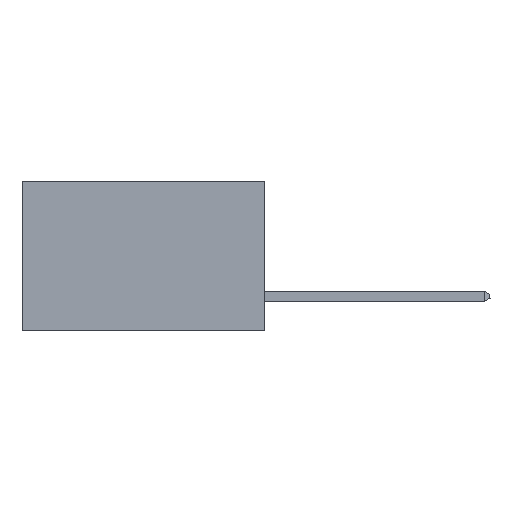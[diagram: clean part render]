
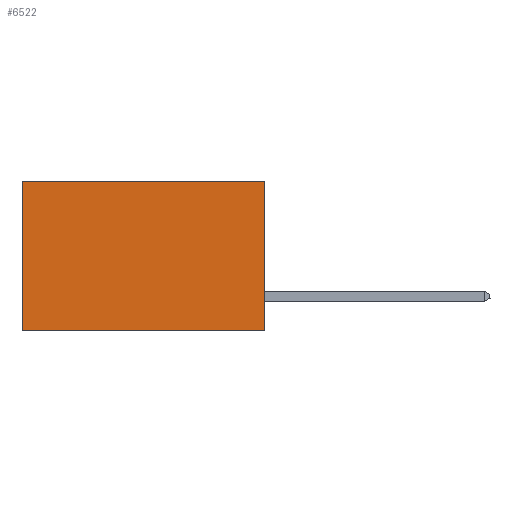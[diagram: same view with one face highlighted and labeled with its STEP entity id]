
A CAD part, left-side view. The second image highlights one B-rep face of the part: STEP entity #6522.
In plain terms, the highlighted planar face has unit normal (-1, 0, 0).
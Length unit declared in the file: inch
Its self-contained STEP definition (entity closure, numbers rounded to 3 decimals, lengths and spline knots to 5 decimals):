
#1373 = DIRECTION ( 'NONE',  ( 0., 0., -1. ) ) ;
#1598 = EDGE_LOOP ( 'NONE', ( #4320, #15465, #14877, #7371 ) ) ;
#2103 = LINE ( 'NONE', #6862, #7607 ) ;
#2368 = EDGE_CURVE ( 'NONE', #15972, #12941, #12220, .T. ) ;
#4251 = CARTESIAN_POINT ( 'NONE',  ( 0.298, 0., 0. ) ) ;
#4320 = ORIENTED_EDGE ( 'NONE', *, *, #8953, .T. ) ;
#4504 = DIRECTION ( 'NONE',  ( 0., 1., 0. ) ) ;
#4635 = CARTESIAN_POINT ( 'NONE',  ( 0.298, 0., -0.37 ) ) ;
#5069 = VECTOR ( 'NONE', #1373, 39.37008 ) ;
#6522 = ADVANCED_FACE ( 'NONE', ( #10808 ), #11775, .F. ) ;
#6862 = CARTESIAN_POINT ( 'NONE',  ( 0.298, 0.6, 0. ) ) ;
#7058 = DIRECTION ( 'NONE',  ( 0., 0., -1. ) ) ;
#7371 = ORIENTED_EDGE ( 'NONE', *, *, #17903, .T. ) ;
#7607 = VECTOR ( 'NONE', #7058, 39.37008 ) ;
#7688 = CARTESIAN_POINT ( 'NONE',  ( 0.298, 0., 0. ) ) ;
#8378 = CARTESIAN_POINT ( 'NONE',  ( 0.298, 0.6, -0.37 ) ) ;
#8698 = LINE ( 'NONE', #7688, #11308 ) ;
#8953 = EDGE_CURVE ( 'NONE', #11469, #17204, #2103, .T. ) ;
#9447 = LINE ( 'NONE', #4635, #12777 ) ;
#10087 = AXIS2_PLACEMENT_3D ( 'NONE', #15025, #18099, #13462 ) ;
#10808 = FACE_OUTER_BOUND ( 'NONE', #1598, .T. ) ;
#11308 = VECTOR ( 'NONE', #18689, 39.37008 ) ;
#11469 = VERTEX_POINT ( 'NONE', #19422 ) ;
#11775 = PLANE ( 'NONE',  #10087 ) ;
#12220 = LINE ( 'NONE', #4251, #5069 ) ;
#12777 = VECTOR ( 'NONE', #4504, 39.37008 ) ;
#12941 = VERTEX_POINT ( 'NONE', #16645 ) ;
#13315 = CARTESIAN_POINT ( 'NONE',  ( 0.298, 0., 0. ) ) ;
#13462 = DIRECTION ( 'NONE',  ( 0., 0., -1. ) ) ;
#14877 = ORIENTED_EDGE ( 'NONE', *, *, #2368, .F. ) ;
#15025 = CARTESIAN_POINT ( 'NONE',  ( 0.298, 0., 0. ) ) ;
#15465 = ORIENTED_EDGE ( 'NONE', *, *, #16575, .F. ) ;
#15972 = VERTEX_POINT ( 'NONE', #13315 ) ;
#16575 = EDGE_CURVE ( 'NONE', #12941, #17204, #9447, .T. ) ;
#16645 = CARTESIAN_POINT ( 'NONE',  ( 0.298, 0., -0.37 ) ) ;
#17204 = VERTEX_POINT ( 'NONE', #8378 ) ;
#17903 = EDGE_CURVE ( 'NONE', #15972, #11469, #8698, .T. ) ;
#18099 = DIRECTION ( 'NONE',  ( 1., 0., 0. ) ) ;
#18689 = DIRECTION ( 'NONE',  ( 0., 1., 0. ) ) ;
#19422 = CARTESIAN_POINT ( 'NONE',  ( 0.298, 0.6, 0. ) ) ;
